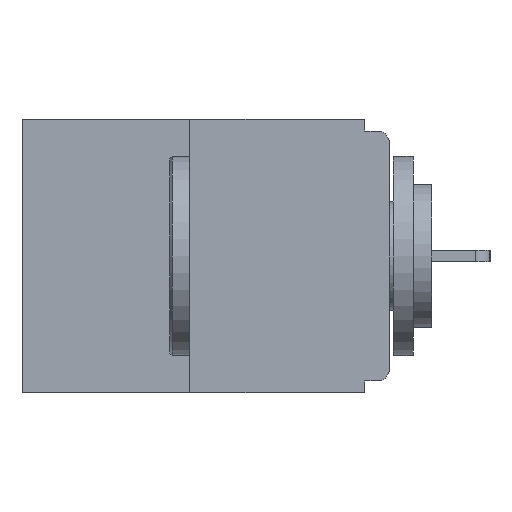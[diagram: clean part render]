
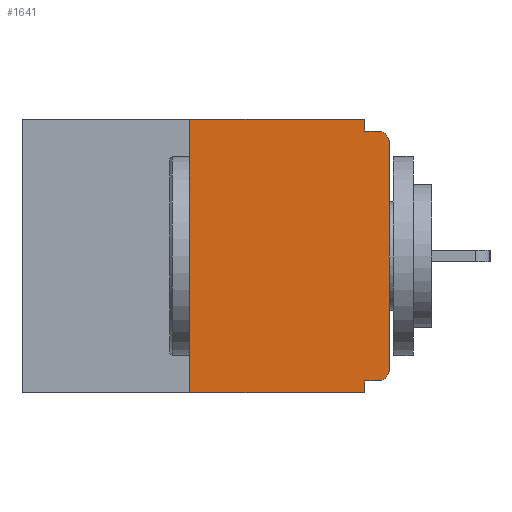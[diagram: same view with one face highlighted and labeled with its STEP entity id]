
A CAD part, left-side view. The second image highlights one B-rep face of the part: STEP entity #1641.
In plain terms, the highlighted planar face has unit normal (-1, 0, 0).
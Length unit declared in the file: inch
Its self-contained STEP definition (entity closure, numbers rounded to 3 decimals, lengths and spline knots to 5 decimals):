
#103 = LINE ( 'NONE', #7313, #11652 ) ;
#572 = EDGE_CURVE ( 'NONE', #12554, #13593, #103, .T. ) ;
#703 = CARTESIAN_POINT ( 'NONE',  ( 0., 0., 0. ) ) ;
#962 = CARTESIAN_POINT ( 'NONE',  ( 0., 0.031, 0. ) ) ;
#1004 = VERTEX_POINT ( 'NONE', #5142 ) ;
#1336 = CARTESIAN_POINT ( 'NONE',  ( 0., 0.015, -0.313 ) ) ;
#1641 = ADVANCED_FACE ( 'NONE', ( #9287 ), #5518, .F. ) ;
#1732 = DIRECTION ( 'NONE',  ( 0., 0., -1. ) ) ;
#1916 = LINE ( 'NONE', #21787, #23308 ) ;
#2993 = LINE ( 'NONE', #12111, #9930 ) ;
#3123 = CIRCLE ( 'NONE', #4641, 0.015 ) ;
#3807 = DIRECTION ( 'NONE',  ( 0., -1., 0. ) ) ;
#3928 = VECTOR ( 'NONE', #4506, 39.37008 ) ;
#4156 = CARTESIAN_POINT ( 'NONE',  ( 0., 0.031, -0.015 ) ) ;
#4167 = ORIENTED_EDGE ( 'NONE', *, *, #572, .F. ) ;
#4328 = LINE ( 'NONE', #9776, #10360 ) ;
#4395 = CARTESIAN_POINT ( 'NONE',  ( 0., 0.015, -0.328 ) ) ;
#4506 = DIRECTION ( 'NONE',  ( 0., 0., 1. ) ) ;
#4641 = AXIS2_PLACEMENT_3D ( 'NONE', #5174, #19619, #16392 ) ;
#5027 = ORIENTED_EDGE ( 'NONE', *, *, #17572, .F. ) ;
#5142 = CARTESIAN_POINT ( 'NONE',  ( 0., 0., -0.313 ) ) ;
#5174 = CARTESIAN_POINT ( 'NONE',  ( 0., 0.015, -0.03 ) ) ;
#5389 = VECTOR ( 'NONE', #1732, 39.37008 ) ;
#5518 = PLANE ( 'NONE',  #8939 ) ;
#5759 = DIRECTION ( 'NONE',  ( 0., -1., 0. ) ) ;
#6025 = CARTESIAN_POINT ( 'NONE',  ( 0., 0.25, 0. ) ) ;
#6110 = EDGE_CURVE ( 'NONE', #16465, #7930, #19910, .T. ) ;
#6140 = LINE ( 'NONE', #15046, #6225 ) ;
#6225 = VECTOR ( 'NONE', #22327, 39.37008 ) ;
#6351 = ORIENTED_EDGE ( 'NONE', *, *, #12718, .T. ) ;
#6440 = DIRECTION ( 'NONE',  ( -1., 0., 0. ) ) ;
#6490 = LINE ( 'NONE', #703, #3928 ) ;
#7313 = CARTESIAN_POINT ( 'NONE',  ( 0., 0., -0.328 ) ) ;
#7320 = ORIENTED_EDGE ( 'NONE', *, *, #20637, .F. ) ;
#7368 = CARTESIAN_POINT ( 'NONE',  ( 0., 0.25, -0.343 ) ) ;
#7554 = VERTEX_POINT ( 'NONE', #962 ) ;
#7694 = VERTEX_POINT ( 'NONE', #4156 ) ;
#7930 = VERTEX_POINT ( 'NONE', #14421 ) ;
#8167 = EDGE_CURVE ( 'NONE', #13593, #7930, #2993, .T. ) ;
#8597 = ORIENTED_EDGE ( 'NONE', *, *, #14127, .T. ) ;
#8874 = DIRECTION ( 'NONE',  ( 0., 0., 1. ) ) ;
#8939 = AXIS2_PLACEMENT_3D ( 'NONE', #18560, #12773, #19977 ) ;
#9034 = CARTESIAN_POINT ( 'NONE',  ( 0., 0.015, -0.015 ) ) ;
#9287 = FACE_OUTER_BOUND ( 'NONE', #16754, .T. ) ;
#9776 = CARTESIAN_POINT ( 'NONE',  ( 0., 0., -0.015 ) ) ;
#9930 = VECTOR ( 'NONE', #14128, 39.37008 ) ;
#9931 = ORIENTED_EDGE ( 'NONE', *, *, #6110, .T. ) ;
#10089 = VERTEX_POINT ( 'NONE', #14232 ) ;
#10360 = VECTOR ( 'NONE', #5759, 39.37008 ) ;
#10748 = LINE ( 'NONE', #17978, #5389 ) ;
#11652 = VECTOR ( 'NONE', #19418, 39.37008 ) ;
#12111 = CARTESIAN_POINT ( 'NONE',  ( 0., 0.031, -0.343 ) ) ;
#12554 = VERTEX_POINT ( 'NONE', #4395 ) ;
#12718 = EDGE_CURVE ( 'NONE', #10089, #18455, #3123, .T. ) ;
#12773 = DIRECTION ( 'NONE',  ( 1., 0., 0. ) ) ;
#13053 = EDGE_CURVE ( 'NONE', #7554, #7694, #10748, .T. ) ;
#13593 = VERTEX_POINT ( 'NONE', #18633 ) ;
#14127 = EDGE_CURVE ( 'NONE', #1004, #10089, #6490, .T. ) ;
#14128 = DIRECTION ( 'NONE',  ( 0., 0., -1. ) ) ;
#14232 = CARTESIAN_POINT ( 'NONE',  ( 0., 0., -0.03 ) ) ;
#14421 = CARTESIAN_POINT ( 'NONE',  ( 0., 0.031, -0.343 ) ) ;
#15046 = CARTESIAN_POINT ( 'NONE',  ( 0., 0.46, 0. ) ) ;
#15494 = AXIS2_PLACEMENT_3D ( 'NONE', #1336, #6440, #17348 ) ;
#15984 = ORIENTED_EDGE ( 'NONE', *, *, #19797, .F. ) ;
#16299 = EDGE_CURVE ( 'NONE', #12554, #1004, #18523, .T. ) ;
#16392 = DIRECTION ( 'NONE',  ( 0., 0., -1. ) ) ;
#16465 = VERTEX_POINT ( 'NONE', #7368 ) ;
#16754 = EDGE_LOOP ( 'NONE', ( #7320, #5027, #9931, #17957, #4167, #17736, #8597, #6351, #15984, #21894 ) ) ;
#17348 = DIRECTION ( 'NONE',  ( 0., 0., -1. ) ) ;
#17572 = EDGE_CURVE ( 'NONE', #16465, #21723, #1916, .T. ) ;
#17736 = ORIENTED_EDGE ( 'NONE', *, *, #16299, .T. ) ;
#17957 = ORIENTED_EDGE ( 'NONE', *, *, #8167, .F. ) ;
#17978 = CARTESIAN_POINT ( 'NONE',  ( 0., 0.031, 0. ) ) ;
#18455 = VERTEX_POINT ( 'NONE', #9034 ) ;
#18523 = CIRCLE ( 'NONE', #15494, 0.015 ) ;
#18560 = CARTESIAN_POINT ( 'NONE',  ( 0., 0.46, 0. ) ) ;
#18633 = CARTESIAN_POINT ( 'NONE',  ( 0., 0.031, -0.328 ) ) ;
#19418 = DIRECTION ( 'NONE',  ( 0., 1., 0. ) ) ;
#19619 = DIRECTION ( 'NONE',  ( -1., 0., 0. ) ) ;
#19797 = EDGE_CURVE ( 'NONE', #7694, #18455, #4328, .T. ) ;
#19910 = LINE ( 'NONE', #21782, #20030 ) ;
#19977 = DIRECTION ( 'NONE',  ( 0., 0., -1. ) ) ;
#20030 = VECTOR ( 'NONE', #3807, 39.37008 ) ;
#20637 = EDGE_CURVE ( 'NONE', #21723, #7554, #6140, .T. ) ;
#21723 = VERTEX_POINT ( 'NONE', #6025 ) ;
#21782 = CARTESIAN_POINT ( 'NONE',  ( 0., 0.46, -0.343 ) ) ;
#21787 = CARTESIAN_POINT ( 'NONE',  ( 0., 0.25, 0. ) ) ;
#21894 = ORIENTED_EDGE ( 'NONE', *, *, #13053, .F. ) ;
#22327 = DIRECTION ( 'NONE',  ( 0., -1., 0. ) ) ;
#23308 = VECTOR ( 'NONE', #8874, 39.37008 ) ;
